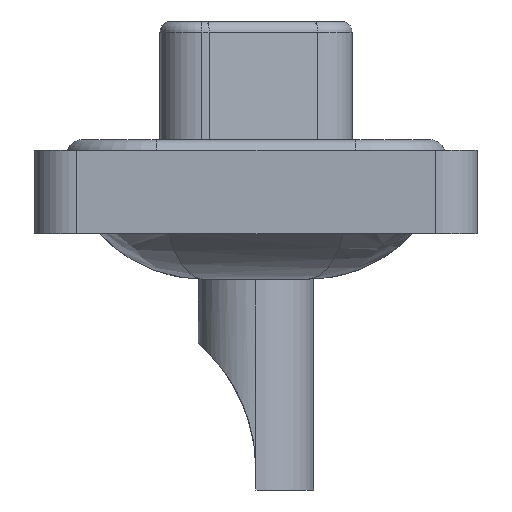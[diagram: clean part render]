
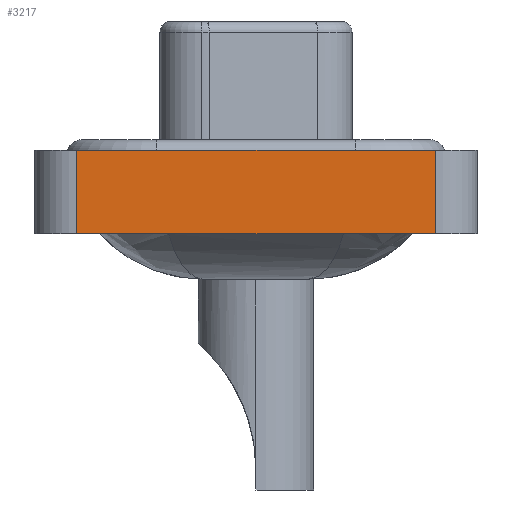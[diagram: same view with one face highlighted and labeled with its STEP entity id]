
A CAD part, left-side view. The second image highlights one B-rep face of the part: STEP entity #3217.
In plain terms, the highlighted planar face has unit normal (-1, 0, 0).
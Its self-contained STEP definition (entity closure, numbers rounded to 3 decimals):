
#260 = VERTEX_POINT ( 'NONE', #16519 ) ;
#1020 = FACE_OUTER_BOUND ( 'NONE', #2761, .T. ) ;
#1231 = DIRECTION ( 'NONE',  ( -1., 0., 0. ) ) ;
#1799 = VERTEX_POINT ( 'NONE', #6867 ) ;
#2751 = DIRECTION ( 'NONE',  ( 0., 0., 1. ) ) ;
#2761 = EDGE_LOOP ( 'NONE', ( #20465, #5787, #9412, #14156 ) ) ;
#2780 = EDGE_CURVE ( 'NONE', #18604, #260, #4357, .T. ) ;
#2936 = DIRECTION ( 'NONE',  ( 0., 0., 1. ) ) ;
#3217 = ADVANCED_FACE ( 'NONE', ( #1020 ), #15695, .T. ) ;
#3408 = EDGE_CURVE ( 'NONE', #18774, #1799, #17893, .T. ) ;
#3756 = CARTESIAN_POINT ( 'NONE',  ( -7.35, 8.55, -3.6 ) ) ;
#4357 = LINE ( 'NONE', #10834, #4456 ) ;
#4456 = VECTOR ( 'NONE', #2751, 1000. ) ;
#4646 = VECTOR ( 'NONE', #8023, 1000. ) ;
#5272 = EDGE_CURVE ( 'NONE', #18604, #18774, #18396, .T. ) ;
#5409 = LINE ( 'NONE', #11909, #20447 ) ;
#5787 = ORIENTED_EDGE ( 'NONE', *, *, #7888, .F. ) ;
#6867 = CARTESIAN_POINT ( 'NONE',  ( -7.35, -8.55, 0.4 ) ) ;
#7888 = EDGE_CURVE ( 'NONE', #260, #1799, #5409, .T. ) ;
#8023 = DIRECTION ( 'NONE',  ( 0., 0., 1. ) ) ;
#8716 = CARTESIAN_POINT ( 'NONE',  ( -7.35, -8.55, -3.6 ) ) ;
#9412 = ORIENTED_EDGE ( 'NONE', *, *, #2780, .F. ) ;
#10834 = CARTESIAN_POINT ( 'NONE',  ( -7.35, 8.55, -3.6 ) ) ;
#11909 = CARTESIAN_POINT ( 'NONE',  ( -7.35, -8.55, 0.4 ) ) ;
#12791 = AXIS2_PLACEMENT_3D ( 'NONE', #15490, #1231, #2936 ) ;
#13147 = CARTESIAN_POINT ( 'NONE',  ( -7.35, -8.55, -3.6 ) ) ;
#13660 = CARTESIAN_POINT ( 'NONE',  ( -7.35, -8.55, -3.6 ) ) ;
#14156 = ORIENTED_EDGE ( 'NONE', *, *, #5272, .T. ) ;
#15490 = CARTESIAN_POINT ( 'NONE',  ( -7.35, -8.55, -3.6 ) ) ;
#15695 = PLANE ( 'NONE',  #12791 ) ;
#16519 = CARTESIAN_POINT ( 'NONE',  ( -7.35, 8.55, 0.4 ) ) ;
#17893 = LINE ( 'NONE', #13147, #4646 ) ;
#18354 = DIRECTION ( 'NONE',  ( 0., -1., 0. ) ) ;
#18396 = LINE ( 'NONE', #8716, #18440 ) ;
#18440 = VECTOR ( 'NONE', #19783, 1000. ) ;
#18604 = VERTEX_POINT ( 'NONE', #3756 ) ;
#18774 = VERTEX_POINT ( 'NONE', #13660 ) ;
#19783 = DIRECTION ( 'NONE',  ( 0., -1., 0. ) ) ;
#20447 = VECTOR ( 'NONE', #18354, 1000. ) ;
#20465 = ORIENTED_EDGE ( 'NONE', *, *, #3408, .T. ) ;
